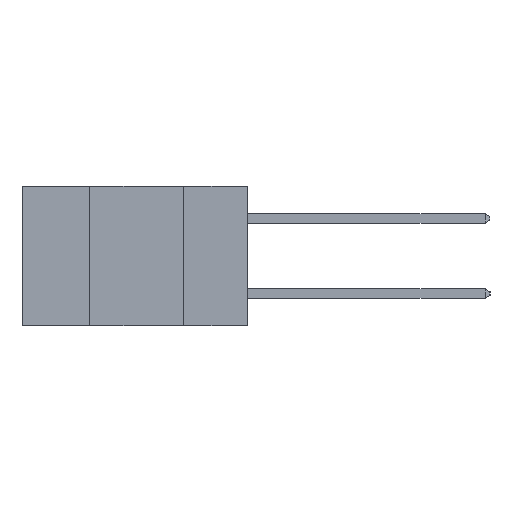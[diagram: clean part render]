
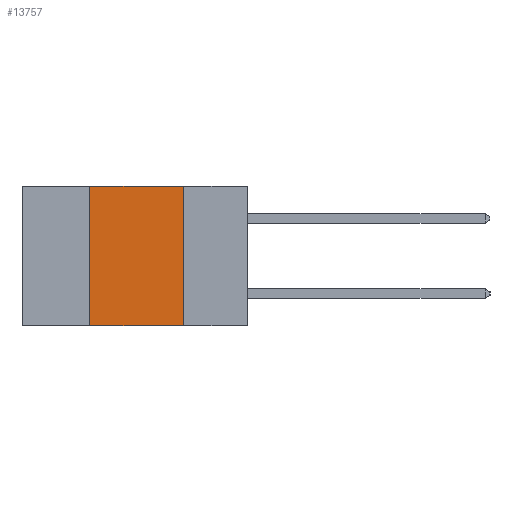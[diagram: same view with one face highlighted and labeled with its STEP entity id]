
A CAD part, left-side view. The second image highlights one B-rep face of the part: STEP entity #13757.
In plain terms, the highlighted planar face has unit normal (-1, 0, 0).
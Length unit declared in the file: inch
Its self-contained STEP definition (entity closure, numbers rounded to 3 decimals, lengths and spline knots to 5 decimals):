
#772 = EDGE_LOOP ( 'NONE', ( #5832, #12416, #17268, #9525 ) ) ;
#1615 = EDGE_CURVE ( 'NONE', #11653, #3926, #1755, .T. ) ;
#1755 = LINE ( 'NONE', #18438, #18416 ) ;
#2036 = VECTOR ( 'NONE', #10912, 39.37008 ) ;
#3351 = LINE ( 'NONE', #9775, #15658 ) ;
#3926 = VERTEX_POINT ( 'NONE', #17166 ) ;
#4455 = CARTESIAN_POINT ( 'NONE',  ( 0., 0.6, 0. ) ) ;
#5832 = ORIENTED_EDGE ( 'NONE', *, *, #1615, .F. ) ;
#6181 = DIRECTION ( 'NONE',  ( 0., 0., -1. ) ) ;
#7787 = CARTESIAN_POINT ( 'NONE',  ( 0., 0.42, -0.37 ) ) ;
#8912 = CARTESIAN_POINT ( 'NONE',  ( 0., 0.6, 0. ) ) ;
#9525 = ORIENTED_EDGE ( 'NONE', *, *, #21447, .T. ) ;
#9775 = CARTESIAN_POINT ( 'NONE',  ( 0., 0.42, -0.37 ) ) ;
#10912 = DIRECTION ( 'NONE',  ( 0., -1., 0. ) ) ;
#11653 = VERTEX_POINT ( 'NONE', #16668 ) ;
#12097 = AXIS2_PLACEMENT_3D ( 'NONE', #4455, #16121, #6181 ) ;
#12301 = DIRECTION ( 'NONE',  ( 0., -1., 0. ) ) ;
#12416 = ORIENTED_EDGE ( 'NONE', *, *, #19318, .F. ) ;
#12700 = VERTEX_POINT ( 'NONE', #7787 ) ;
#12817 = FACE_OUTER_BOUND ( 'NONE', #772, .T. ) ;
#13157 = DIRECTION ( 'NONE',  ( 0., 0., 1. ) ) ;
#13423 = DIRECTION ( 'NONE',  ( 0., 0., -1. ) ) ;
#13757 = ADVANCED_FACE ( 'NONE', ( #12817 ), #14492, .F. ) ;
#14492 = PLANE ( 'NONE',  #12097 ) ;
#15153 = VERTEX_POINT ( 'NONE', #17831 ) ;
#15658 = VECTOR ( 'NONE', #13157, 39.37008 ) ;
#15819 = CARTESIAN_POINT ( 'NONE',  ( 0., 0.6, -0.37 ) ) ;
#15969 = VECTOR ( 'NONE', #12301, 39.37008 ) ;
#16121 = DIRECTION ( 'NONE',  ( 1., 0., 0. ) ) ;
#16668 = CARTESIAN_POINT ( 'NONE',  ( 0., 0.17, 0. ) ) ;
#17166 = CARTESIAN_POINT ( 'NONE',  ( 0., 0.17, -0.37 ) ) ;
#17268 = ORIENTED_EDGE ( 'NONE', *, *, #20387, .F. ) ;
#17831 = CARTESIAN_POINT ( 'NONE',  ( 0., 0.42, 0. ) ) ;
#18416 = VECTOR ( 'NONE', #13423, 39.37008 ) ;
#18438 = CARTESIAN_POINT ( 'NONE',  ( 0., 0.17, -0.37 ) ) ;
#18696 = LINE ( 'NONE', #15819, #2036 ) ;
#19318 = EDGE_CURVE ( 'NONE', #15153, #11653, #20769, .T. ) ;
#20387 = EDGE_CURVE ( 'NONE', #12700, #15153, #3351, .T. ) ;
#20769 = LINE ( 'NONE', #8912, #15969 ) ;
#21447 = EDGE_CURVE ( 'NONE', #12700, #3926, #18696, .T. ) ;
